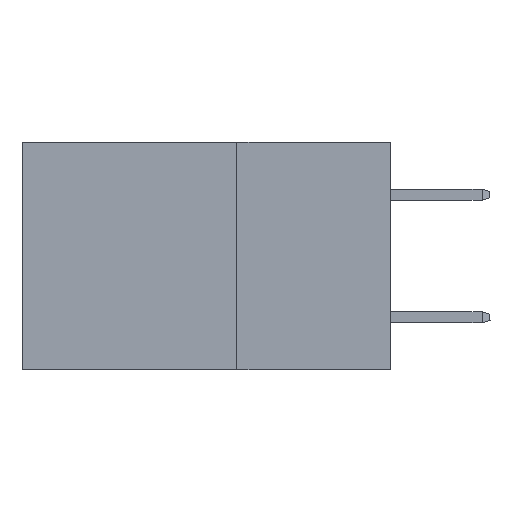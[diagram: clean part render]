
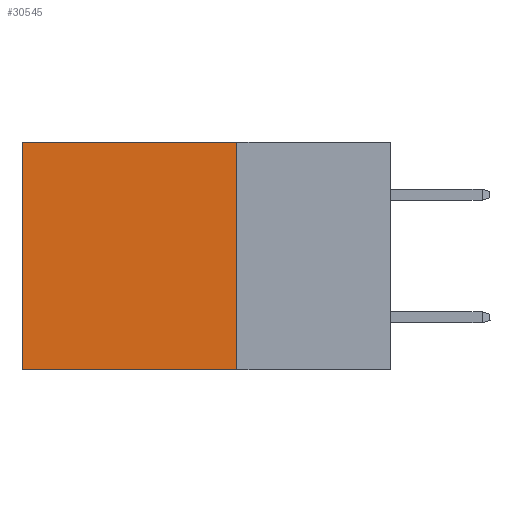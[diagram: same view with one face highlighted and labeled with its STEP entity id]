
A CAD part, left-side view. The second image highlights one B-rep face of the part: STEP entity #30545.
In plain terms, the highlighted planar face has unit normal (-1, 0, 0).
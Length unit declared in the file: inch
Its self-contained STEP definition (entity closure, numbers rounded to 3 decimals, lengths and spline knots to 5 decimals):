
#1119 = DIRECTION ( 'NONE',  ( 0., 0., -1. ) ) ;
#2644 = EDGE_CURVE ( 'NONE', #12803, #24378, #24371, .T. ) ;
#4294 = CARTESIAN_POINT ( 'NONE',  ( 0.2875, 0.6, 0. ) ) ;
#5875 = EDGE_CURVE ( 'NONE', #32351, #12803, #39623, .T. ) ;
#6944 = VECTOR ( 'NONE', #1119, 39.37008 ) ;
#7935 = LINE ( 'NONE', #38889, #6944 ) ;
#8991 = EDGE_LOOP ( 'NONE', ( #11464, #16596, #14352, #27769 ) ) ;
#11464 = ORIENTED_EDGE ( 'NONE', *, *, #25437, .T. ) ;
#12803 = VERTEX_POINT ( 'NONE', #32793 ) ;
#13310 = CARTESIAN_POINT ( 'NONE',  ( 0.2875, 0.25, 0. ) ) ;
#13847 = DIRECTION ( 'NONE',  ( 0., 1., 0. ) ) ;
#14352 = ORIENTED_EDGE ( 'NONE', *, *, #5875, .F. ) ;
#14400 = VECTOR ( 'NONE', #21795, 39.37008 ) ;
#16596 = ORIENTED_EDGE ( 'NONE', *, *, #2644, .F. ) ;
#16969 = PLANE ( 'NONE',  #37406 ) ;
#18730 = LINE ( 'NONE', #13310, #26116 ) ;
#20545 = DIRECTION ( 'NONE',  ( 1., 0., 0. ) ) ;
#21050 = CARTESIAN_POINT ( 'NONE',  ( 0.2875, 0.6, -0.37 ) ) ;
#21795 = DIRECTION ( 'NONE',  ( 0., 0., -1. ) ) ;
#22914 = DIRECTION ( 'NONE',  ( 0., 1., 0. ) ) ;
#24371 = LINE ( 'NONE', #38767, #40146 ) ;
#24378 = VERTEX_POINT ( 'NONE', #21050 ) ;
#25437 = EDGE_CURVE ( 'NONE', #29748, #24378, #7935, .T. ) ;
#26116 = VECTOR ( 'NONE', #13847, 39.37008 ) ;
#27769 = ORIENTED_EDGE ( 'NONE', *, *, #38796, .T. ) ;
#29748 = VERTEX_POINT ( 'NONE', #4294 ) ;
#30545 = ADVANCED_FACE ( 'NONE', ( #38907 ), #16969, .F. ) ;
#31054 = CARTESIAN_POINT ( 'NONE',  ( 0.2875, 0.25, 0. ) ) ;
#31357 = CARTESIAN_POINT ( 'NONE',  ( 0.2875, 0.25, 0. ) ) ;
#32351 = VERTEX_POINT ( 'NONE', #31357 ) ;
#32793 = CARTESIAN_POINT ( 'NONE',  ( 0.2875, 0.25, -0.37 ) ) ;
#32956 = DIRECTION ( 'NONE',  ( 0., 0., -1. ) ) ;
#33082 = CARTESIAN_POINT ( 'NONE',  ( 0.2875, 0.25, 0. ) ) ;
#37406 = AXIS2_PLACEMENT_3D ( 'NONE', #33082, #20545, #32956 ) ;
#38767 = CARTESIAN_POINT ( 'NONE',  ( 0.2875, 0.25, -0.37 ) ) ;
#38796 = EDGE_CURVE ( 'NONE', #32351, #29748, #18730, .T. ) ;
#38889 = CARTESIAN_POINT ( 'NONE',  ( 0.2875, 0.6, 0. ) ) ;
#38907 = FACE_OUTER_BOUND ( 'NONE', #8991, .T. ) ;
#39623 = LINE ( 'NONE', #31054, #14400 ) ;
#40146 = VECTOR ( 'NONE', #22914, 39.37008 ) ;
